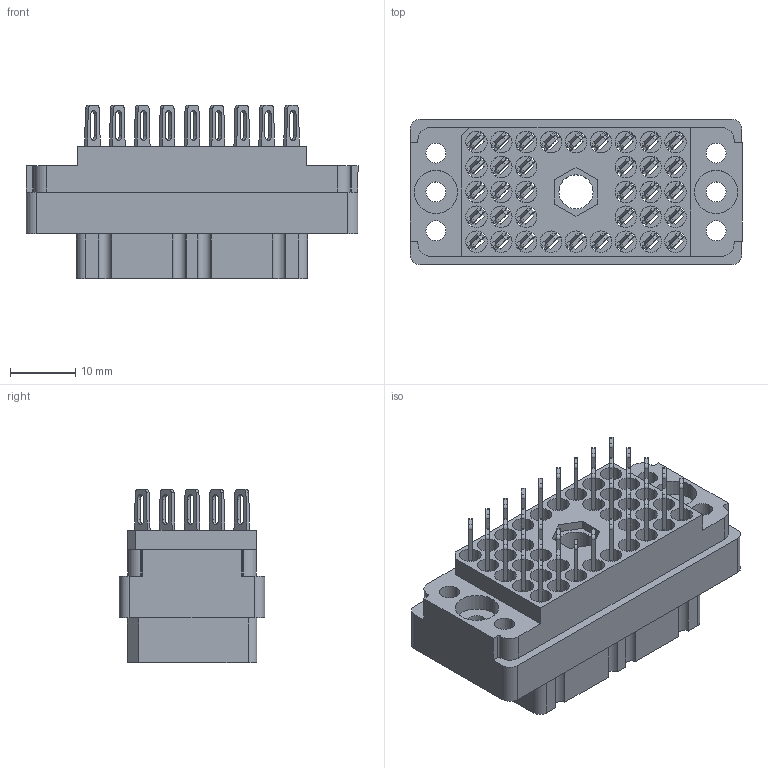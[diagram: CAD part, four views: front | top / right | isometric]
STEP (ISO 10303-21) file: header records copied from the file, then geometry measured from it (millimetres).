
FILE_DESCRIPTION (( 'STEP AP203' ), '1' );
FILE_NAME ('519-036-500-400.STEP', '2020-09-09T20:10:55', ( '' ), ( '' ), 'SwSTEP 2.0', 'SolidWorks 2020', '' );
FILE_SCHEMA (( 'CONFIG_CONTROL_DESIGN' ));
Length unit declared in the file: inch
Products named in the file (3): 516-292-001_500 Contact; 519-036-500-400; 519 Receptacle Insulator_036
Assembly tree (37 placements, depth 2):
  519-036-500-400
    519 Receptacle Insulator_036
    516-292-001_500 Contact  x36
Bounding box: 50.8 x 22.25 x 26.49 mm (x, y, z)
Volume: 12429.1 mm3; surface area: 20592.5 mm2
Topology: 37 solids, 37 shells, 3583 faces, 10403 edges, 6910 vertices
Faces by surface type: plane 2159, cylinder 1206, bspline 216, cone 2
Entity records: 32409 total; most frequent: CARTESIAN_POINT 5751, ORIENTED_EDGE 5406, DIRECTION 5241, EDGE_CURVE 2703, VECTOR 2011, LINE 2011, VERTEX_POINT 1800, AXIS2_PLACEMENT_3D 1615
